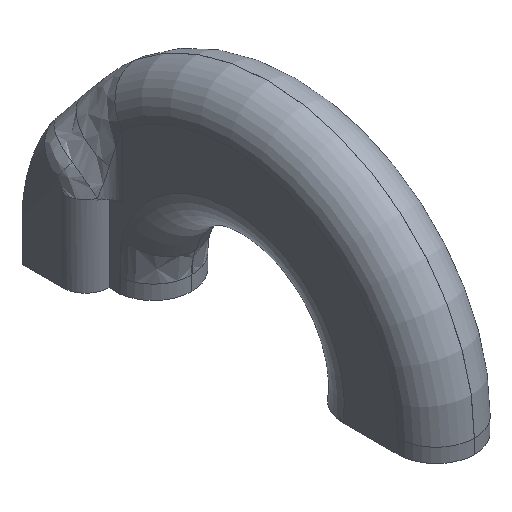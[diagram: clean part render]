
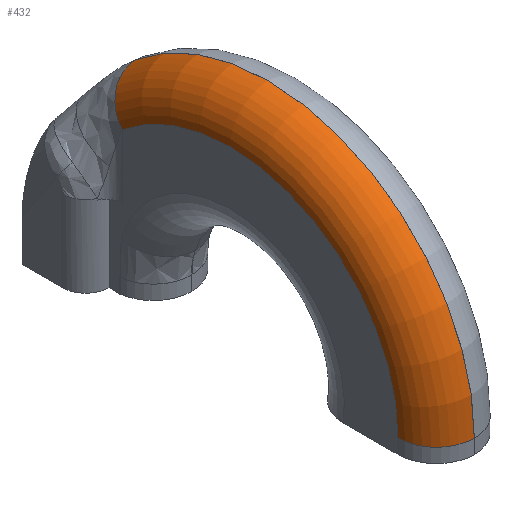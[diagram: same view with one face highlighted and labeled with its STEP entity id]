
A CAD part, isometric view. The second image highlights one B-rep face of the part: STEP entity #432.
In plain terms, the highlighted toroidal (fillet/blend) face has major radius 50.7 mm and minor radius 11.5 mm.
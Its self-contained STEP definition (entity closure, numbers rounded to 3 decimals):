
#12 = DIRECTION ( 'NONE',  ( 0., 0.641, 0.767 ) ) ;
#15 = DIRECTION ( 'NONE',  ( 0., 0.767, -0.641 ) ) ;
#16 = CARTESIAN_POINT ( 'NONE',  ( -75.573, 22.63, 22.729 ) ) ;
#23 = DIRECTION ( 'NONE',  ( 1., 0., 0. ) ) ;
#35 = DIRECTION ( 'NONE',  ( 0., 0., -1. ) ) ;
#45 = CARTESIAN_POINT ( 'NONE',  ( -75.573, -9.877, -16.179 ) ) ;
#91 = CARTESIAN_POINT ( 'NONE',  ( -87.073, 22.63, 22.729 ) ) ;
#190 = CARTESIAN_POINT ( 'NONE',  ( -75.573, 30.003, 31.554 ) ) ;
#235 = AXIS2_PLACEMENT_3D ( 'NONE', #827, #972, #819 ) ;
#338 = DIRECTION ( 'NONE',  ( 1., 0., 0. ) ) ;
#341 = CARTESIAN_POINT ( 'NONE',  ( -75.573, -60.577, -16.179 ) ) ;
#352 = DIRECTION ( 'NONE',  ( 0., 0., 1. ) ) ;
#432 = ADVANCED_FACE ( 'NONE', ( #1036 ), #1034, .T. ) ;
#565 = AXIS2_PLACEMENT_3D ( 'NONE', #2094, #2092, #2089 ) ;
#587 = AXIS2_PLACEMENT_3D ( 'NONE', #45, #23, #35 ) ;
#599 = AXIS2_PLACEMENT_3D ( 'NONE', #341, #352, #338 ) ;
#601 = CARTESIAN_POINT ( 'NONE',  ( -87.073, -60.577, -16.179 ) ) ;
#636 = CARTESIAN_POINT ( 'NONE',  ( -75.573, -72.077, -16.179 ) ) ;
#694 = AXIS2_PLACEMENT_3D ( 'NONE', #16, #15, #12 ) ;
#797 = CIRCLE ( 'NONE', #565, 50.7 ) ;
#816 = CIRCLE ( 'NONE', #587, 62.2 ) ;
#819 = DIRECTION ( 'NONE',  ( 0., 0., -1. ) ) ;
#824 = CIRCLE ( 'NONE', #599, 11.5 ) ;
#827 = CARTESIAN_POINT ( 'NONE',  ( -75.573, -9.877, -16.179 ) ) ;
#922 = CIRCLE ( 'NONE', #694, 11.5 ) ;
#972 = DIRECTION ( 'NONE',  ( 1., 0., 0. ) ) ;
#1034 = TOROIDAL_SURFACE ( 'NONE', #235, 50.7, 11.5 ) ;
#1036 = FACE_OUTER_BOUND ( 'NONE', #1252, .T. ) ;
#1252 = EDGE_LOOP ( 'NONE', ( #1834, #1828, #2076, #1418 ) ) ;
#1273 = VERTEX_POINT ( 'NONE', #636 ) ;
#1418 = ORIENTED_EDGE ( 'NONE', *, *, #2021, .F. ) ;
#1461 = VERTEX_POINT ( 'NONE', #601 ) ;
#1570 = VERTEX_POINT ( 'NONE', #190 ) ;
#1651 = VERTEX_POINT ( 'NONE', #91 ) ;
#1685 = EDGE_CURVE ( 'NONE', #1651, #1570, #922, .T. ) ;
#1828 = ORIENTED_EDGE ( 'NONE', *, *, #1934, .F. ) ;
#1834 = ORIENTED_EDGE ( 'NONE', *, *, #1898, .T. ) ;
#1898 = EDGE_CURVE ( 'NONE', #1461, #1273, #824, .T. ) ;
#1934 = EDGE_CURVE ( 'NONE', #1570, #1273, #816, .T. ) ;
#2021 = EDGE_CURVE ( 'NONE', #1461, #1651, #797, .T. ) ;
#2076 = ORIENTED_EDGE ( 'NONE', *, *, #1685, .F. ) ;
#2089 = DIRECTION ( 'NONE',  ( 0., 0., -1. ) ) ;
#2092 = DIRECTION ( 'NONE',  ( -1., 0., 0. ) ) ;
#2094 = CARTESIAN_POINT ( 'NONE',  ( -87.073, -9.877, -16.179 ) ) ;
